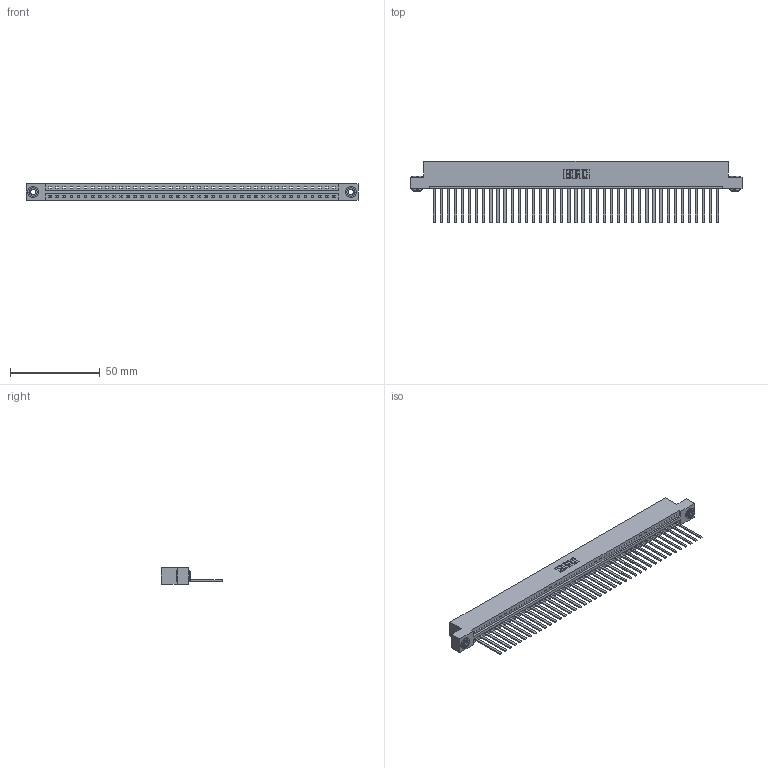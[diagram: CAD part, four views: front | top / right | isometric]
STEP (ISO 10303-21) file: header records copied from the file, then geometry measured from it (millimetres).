
FILE_DESCRIPTION (( 'STEP AP203' ), '1' );
FILE_NAME ('387-041-544-103.STEP', '2019-10-04T20:09:11', ( '' ), ( '' ), 'SwSTEP 2.0', 'SolidWorks 2016', '' );
FILE_SCHEMA (( 'CONFIG_CONTROL_DESIGN' ));
Length unit declared in the file: inch
Products named in the file (4): 345-250-002_345-250-002-102; 345-292-001_345-293-144; 387-041-544-103; 337 Part_Flush Mounting Lugs - 0.156 Dia-TH
Assembly tree (44 placements, depth 2):
  387-041-544-103
    337 Part_Flush Mounting Lugs - 0.156 Dia-TH
    345-292-001_345-293-144  x41
    345-250-002_345-250-002-102  x2
Bounding box: 185.47 x 34.3 x 9.4 mm (x, y, z)
Volume: 19758.3 mm3; surface area: 22206.4 mm2
Topology: 44 solids, 44 shells, 2448 faces, 7357 edges, 4846 vertices
Faces by surface type: plane 1802, cylinder 638, cone 8
Entity records: 31072 total; most frequent: CARTESIAN_POINT 5388, ORIENTED_EDGE 5358, DIRECTION 4567, EDGE_CURVE 2679, VECTOR 2531, LINE 2531, VERTEX_POINT 1782, AXIS2_PLACEMENT_3D 1018
